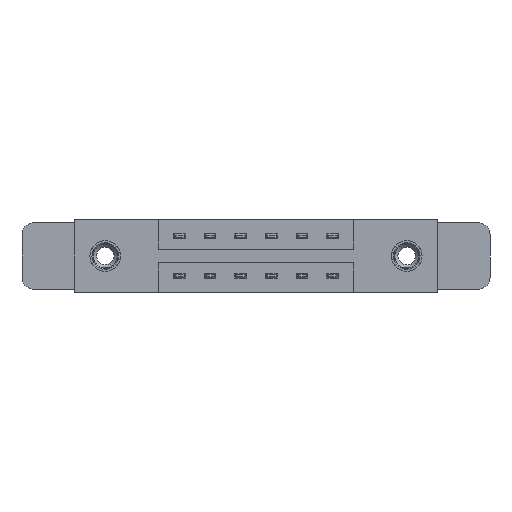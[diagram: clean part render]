
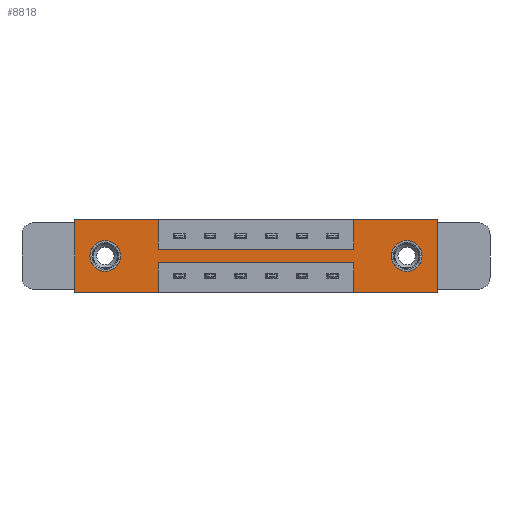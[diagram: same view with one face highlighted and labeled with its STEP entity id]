
A CAD part, front view. The second image highlights one B-rep face of the part: STEP entity #8818.
In plain terms, the highlighted planar face has unit normal (0, -1, 0).
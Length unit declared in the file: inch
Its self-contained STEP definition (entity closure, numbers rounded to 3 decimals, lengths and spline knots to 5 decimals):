
#20 = CARTESIAN_POINT ( 'NONE',  ( 0.425, 0., -0.22 ) ) ;
#75 = CARTESIAN_POINT ( 'NONE',  ( 0.425, 0., 0. ) ) ;
#377 = ORIENTED_EDGE ( 'NONE', *, *, #4764, .F. ) ;
#393 = VERTEX_POINT ( 'NONE', #11204 ) ;
#444 = DIRECTION ( 'NONE',  ( 0., 1., 0. ) ) ;
#549 = FACE_BOUND ( 'NONE', #10722, .T. ) ;
#588 = DIRECTION ( 'NONE',  ( 0., 0., -1. ) ) ;
#653 = VERTEX_POINT ( 'NONE', #10789 ) ;
#804 = VERTEX_POINT ( 'NONE', #2901 ) ;
#859 = EDGE_CURVE ( 'NONE', #2751, #9627, #2856, .T. ) ;
#1011 = LINE ( 'NONE', #4188, #6025 ) ;
#1026 = LINE ( 'NONE', #3140, #1883 ) ;
#1079 = ORIENTED_EDGE ( 'NONE', *, *, #10558, .T. ) ;
#1133 = CIRCLE ( 'NONE', #6905, 0.078 ) ;
#1338 = EDGE_CURVE ( 'NONE', #393, #9933, #7732, .T. ) ;
#1339 = CARTESIAN_POINT ( 'NONE',  ( 0.155, 0., -0.185 ) ) ;
#1472 = ORIENTED_EDGE ( 'NONE', *, *, #11482, .F. ) ;
#1554 = CARTESIAN_POINT ( 'NONE',  ( 0., 0., 0. ) ) ;
#1882 = CARTESIAN_POINT ( 'NONE',  ( 1.687, 0., -0.107 ) ) ;
#1883 = VECTOR ( 'NONE', #5914, 39.37008 ) ;
#1918 = VERTEX_POINT ( 'NONE', #2026 ) ;
#1939 = CARTESIAN_POINT ( 'NONE',  ( 1.417, 0., -0.37 ) ) ;
#2026 = CARTESIAN_POINT ( 'NONE',  ( 1.417, 0., 0. ) ) ;
#2032 = LINE ( 'NONE', #4818, #9709 ) ;
#2051 = VERTEX_POINT ( 'NONE', #3105 ) ;
#2119 = VERTEX_POINT ( 'NONE', #11220 ) ;
#2183 = DIRECTION ( 'NONE',  ( 0., 0., 1. ) ) ;
#2241 = ORIENTED_EDGE ( 'NONE', *, *, #5850, .T. ) ;
#2541 = DIRECTION ( 'NONE',  ( 0., 0., 1. ) ) ;
#2571 = EDGE_CURVE ( 'NONE', #2051, #4502, #9181, .T. ) ;
#2733 = ORIENTED_EDGE ( 'NONE', *, *, #4577, .F. ) ;
#2751 = VERTEX_POINT ( 'NONE', #4076 ) ;
#2822 = PLANE ( 'NONE',  #3789 ) ;
#2848 = VECTOR ( 'NONE', #10056, 39.37008 ) ;
#2856 = LINE ( 'NONE', #75, #5582 ) ;
#2901 = CARTESIAN_POINT ( 'NONE',  ( 0.425, 0., -0.37 ) ) ;
#2939 = DIRECTION ( 'NONE',  ( 1., 0., 0. ) ) ;
#3089 = DIRECTION ( 'NONE',  ( 0., 0., 1. ) ) ;
#3100 = ORIENTED_EDGE ( 'NONE', *, *, #10509, .F. ) ;
#3105 = CARTESIAN_POINT ( 'NONE',  ( 1.842, 0., -0.37 ) ) ;
#3140 = CARTESIAN_POINT ( 'NONE',  ( 0.425, 0., -0.37 ) ) ;
#3321 = ORIENTED_EDGE ( 'NONE', *, *, #8833, .F. ) ;
#3394 = ORIENTED_EDGE ( 'NONE', *, *, #1338, .F. ) ;
#3480 = VECTOR ( 'NONE', #7469, 39.37008 ) ;
#3512 = EDGE_CURVE ( 'NONE', #9504, #10375, #8469, .T. ) ;
#3653 = DIRECTION ( 'NONE',  ( 0., 1., 0. ) ) ;
#3789 = AXIS2_PLACEMENT_3D ( 'NONE', #4665, #6440, #6605 ) ;
#3832 = VECTOR ( 'NONE', #6289, 39.37008 ) ;
#3836 = CARTESIAN_POINT ( 'NONE',  ( 0., 0., -0.37 ) ) ;
#4076 = CARTESIAN_POINT ( 'NONE',  ( 0.425, 0., 0. ) ) ;
#4095 = EDGE_CURVE ( 'NONE', #9933, #804, #1026, .T. ) ;
#4111 = LINE ( 'NONE', #1554, #4966 ) ;
#4153 = LINE ( 'NONE', #10037, #4717 ) ;
#4164 = DIRECTION ( 'NONE',  ( 0., 0., -1. ) ) ;
#4183 = CARTESIAN_POINT ( 'NONE',  ( 0.425, 0., -0.15 ) ) ;
#4188 = CARTESIAN_POINT ( 'NONE',  ( 1.842, 0., 0. ) ) ;
#4352 = LINE ( 'NONE', #11633, #7353 ) ;
#4474 = ORIENTED_EDGE ( 'NONE', *, *, #4095, .F. ) ;
#4483 = EDGE_LOOP ( 'NONE', ( #1079, #8805 ) ) ;
#4502 = VERTEX_POINT ( 'NONE', #1939 ) ;
#4577 = EDGE_CURVE ( 'NONE', #9627, #653, #2032, .T. ) ;
#4665 = CARTESIAN_POINT ( 'NONE',  ( 0., 0., -0.37 ) ) ;
#4717 = VECTOR ( 'NONE', #9993, 39.37008 ) ;
#4764 = EDGE_CURVE ( 'NONE', #7125, #2051, #1011, .T. ) ;
#4804 = ORIENTED_EDGE ( 'NONE', *, *, #2571, .F. ) ;
#4818 = CARTESIAN_POINT ( 'NONE',  ( 0.425, 0., -0.15 ) ) ;
#4966 = VECTOR ( 'NONE', #7945, 39.37008 ) ;
#4983 = LINE ( 'NONE', #7418, #10515 ) ;
#5001 = CARTESIAN_POINT ( 'NONE',  ( 1.687, 0., -0.185 ) ) ;
#5084 = EDGE_CURVE ( 'NONE', #653, #1918, #4153, .T. ) ;
#5092 = ORIENTED_EDGE ( 'NONE', *, *, #8690, .T. ) ;
#5175 = ORIENTED_EDGE ( 'NONE', *, *, #8706, .F. ) ;
#5194 = CARTESIAN_POINT ( 'NONE',  ( 0.155, 0., -0.263 ) ) ;
#5224 = CIRCLE ( 'NONE', #6439, 0.078 ) ;
#5255 = FACE_BOUND ( 'NONE', #4483, .T. ) ;
#5368 = CARTESIAN_POINT ( 'NONE',  ( 0., 0., 0. ) ) ;
#5395 = FACE_OUTER_BOUND ( 'NONE', #8329, .T. ) ;
#5472 = ORIENTED_EDGE ( 'NONE', *, *, #6857, .F. ) ;
#5519 = LINE ( 'NONE', #8462, #7795 ) ;
#5582 = VECTOR ( 'NONE', #6447, 39.37008 ) ;
#5732 = CARTESIAN_POINT ( 'NONE',  ( 1.687, 0., -0.185 ) ) ;
#5759 = CARTESIAN_POINT ( 'NONE',  ( 0.155, 0., -0.107 ) ) ;
#5850 = EDGE_CURVE ( 'NONE', #6066, #8375, #1133, .T. ) ;
#5914 = DIRECTION ( 'NONE',  ( 0., 0., -1. ) ) ;
#6025 = VECTOR ( 'NONE', #588, 39.37008 ) ;
#6066 = VERTEX_POINT ( 'NONE', #5194 ) ;
#6282 = CIRCLE ( 'NONE', #9045, 0.078 ) ;
#6289 = DIRECTION ( 'NONE',  ( -1., 0., 0. ) ) ;
#6365 = DIRECTION ( 'NONE',  ( 0., 0., 1. ) ) ;
#6439 = AXIS2_PLACEMENT_3D ( 'NONE', #5732, #10325, #8506 ) ;
#6440 = DIRECTION ( 'NONE',  ( 0., -1., 0. ) ) ;
#6447 = DIRECTION ( 'NONE',  ( 0., 0., -1. ) ) ;
#6592 = DIRECTION ( 'NONE',  ( 1., 0., 0. ) ) ;
#6605 = DIRECTION ( 'NONE',  ( 0., 0., -1. ) ) ;
#6735 = CARTESIAN_POINT ( 'NONE',  ( 1.687, 0., -0.263 ) ) ;
#6797 = DIRECTION ( 'NONE',  ( 0., 1., 0. ) ) ;
#6857 = EDGE_CURVE ( 'NONE', #11537, #2751, #4111, .T. ) ;
#6905 = AXIS2_PLACEMENT_3D ( 'NONE', #1339, #6797, #2183 ) ;
#7125 = VERTEX_POINT ( 'NONE', #9356 ) ;
#7353 = VECTOR ( 'NONE', #2541, 39.37008 ) ;
#7410 = AXIS2_PLACEMENT_3D ( 'NONE', #5001, #444, #4164 ) ;
#7418 = CARTESIAN_POINT ( 'NONE',  ( 0., 0., 0. ) ) ;
#7469 = DIRECTION ( 'NONE',  ( -1., 0., 0. ) ) ;
#7732 = LINE ( 'NONE', #20, #2848 ) ;
#7795 = VECTOR ( 'NONE', #3089, 39.37008 ) ;
#7923 = ORIENTED_EDGE ( 'NONE', *, *, #5084, .F. ) ;
#7945 = DIRECTION ( 'NONE',  ( 1., 0., 0. ) ) ;
#8045 = CARTESIAN_POINT ( 'NONE',  ( 0.155, 0., -0.185 ) ) ;
#8237 = ORIENTED_EDGE ( 'NONE', *, *, #859, .F. ) ;
#8329 = EDGE_LOOP ( 'NONE', ( #4474, #3394, #1472, #4804, #377, #3321, #7923, #2733, #8237, #5472, #3100, #5175 ) ) ;
#8375 = VERTEX_POINT ( 'NONE', #5759 ) ;
#8462 = CARTESIAN_POINT ( 'NONE',  ( 0., 0., 0. ) ) ;
#8469 = CIRCLE ( 'NONE', #7410, 0.078 ) ;
#8506 = DIRECTION ( 'NONE',  ( 0., 0., -1. ) ) ;
#8690 = EDGE_CURVE ( 'NONE', #8375, #6066, #6282, .T. ) ;
#8706 = EDGE_CURVE ( 'NONE', #804, #2119, #10090, .T. ) ;
#8805 = ORIENTED_EDGE ( 'NONE', *, *, #3512, .T. ) ;
#8818 = ADVANCED_FACE ( 'NONE', ( #5255, #549, #5395 ), #2822, .T. ) ;
#8833 = EDGE_CURVE ( 'NONE', #1918, #7125, #4983, .T. ) ;
#9045 = AXIS2_PLACEMENT_3D ( 'NONE', #8045, #3653, #6365 ) ;
#9181 = LINE ( 'NONE', #3836, #3480 ) ;
#9356 = CARTESIAN_POINT ( 'NONE',  ( 1.842, 0., 0. ) ) ;
#9504 = VERTEX_POINT ( 'NONE', #6735 ) ;
#9627 = VERTEX_POINT ( 'NONE', #4183 ) ;
#9709 = VECTOR ( 'NONE', #6592, 39.37008 ) ;
#9860 = CARTESIAN_POINT ( 'NONE',  ( 0., 0., -0.37 ) ) ;
#9933 = VERTEX_POINT ( 'NONE', #10288 ) ;
#9993 = DIRECTION ( 'NONE',  ( 0., 0., 1. ) ) ;
#10037 = CARTESIAN_POINT ( 'NONE',  ( 1.417, 0., 0. ) ) ;
#10056 = DIRECTION ( 'NONE',  ( -1., 0., 0. ) ) ;
#10090 = LINE ( 'NONE', #9860, #3832 ) ;
#10288 = CARTESIAN_POINT ( 'NONE',  ( 0.425, 0., -0.22 ) ) ;
#10325 = DIRECTION ( 'NONE',  ( 0., 1., 0. ) ) ;
#10375 = VERTEX_POINT ( 'NONE', #1882 ) ;
#10509 = EDGE_CURVE ( 'NONE', #2119, #11537, #5519, .T. ) ;
#10515 = VECTOR ( 'NONE', #2939, 39.37008 ) ;
#10558 = EDGE_CURVE ( 'NONE', #10375, #9504, #5224, .T. ) ;
#10722 = EDGE_LOOP ( 'NONE', ( #5092, #2241 ) ) ;
#10789 = CARTESIAN_POINT ( 'NONE',  ( 1.417, 0., -0.15 ) ) ;
#11204 = CARTESIAN_POINT ( 'NONE',  ( 1.417, 0., -0.22 ) ) ;
#11220 = CARTESIAN_POINT ( 'NONE',  ( 0., 0., -0.37 ) ) ;
#11482 = EDGE_CURVE ( 'NONE', #4502, #393, #4352, .T. ) ;
#11537 = VERTEX_POINT ( 'NONE', #5368 ) ;
#11633 = CARTESIAN_POINT ( 'NONE',  ( 1.417, 0., -0.37 ) ) ;
